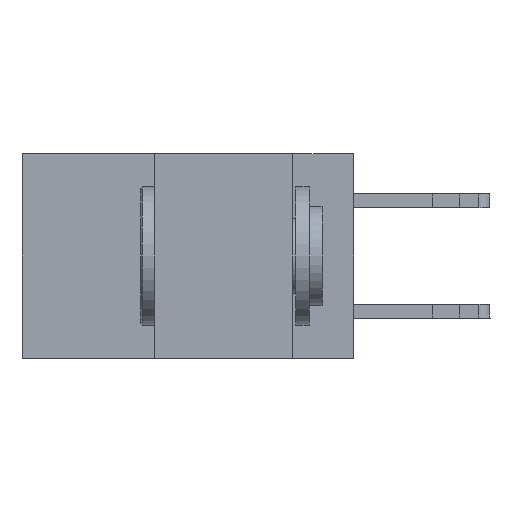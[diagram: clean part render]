
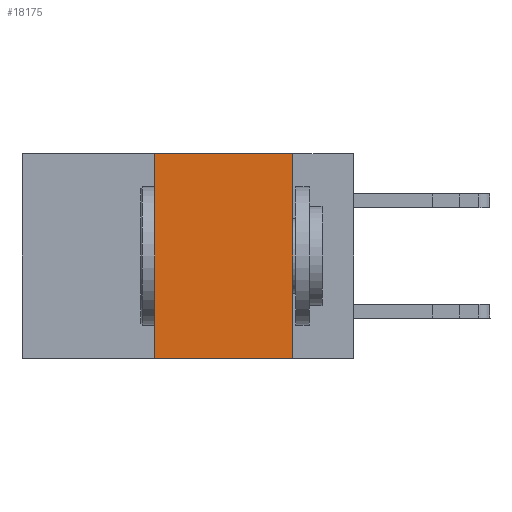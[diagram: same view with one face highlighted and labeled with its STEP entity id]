
A CAD part, left-side view. The second image highlights one B-rep face of the part: STEP entity #18175.
In plain terms, the highlighted planar face has unit normal (-1, 0, 0).
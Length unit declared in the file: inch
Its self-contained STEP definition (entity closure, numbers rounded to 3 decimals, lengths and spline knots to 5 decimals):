
#351 = EDGE_CURVE ( 'NONE', #27454, #6469, #26535, .T. ) ;
#2297 = ORIENTED_EDGE ( 'NONE', *, *, #351, .F. ) ;
#3626 = CARTESIAN_POINT ( 'NONE',  ( 0., 0.11, 0. ) ) ;
#4558 = EDGE_CURVE ( 'NONE', #6469, #20078, #29468, .T. ) ;
#5066 = CARTESIAN_POINT ( 'NONE',  ( 0., 0.36, 0. ) ) ;
#5669 = CARTESIAN_POINT ( 'NONE',  ( 0., 0.11, 0. ) ) ;
#5768 = CARTESIAN_POINT ( 'NONE',  ( 0., 0.6, 0. ) ) ;
#6469 = VERTEX_POINT ( 'NONE', #5669 ) ;
#6593 = LINE ( 'NONE', #22455, #13345 ) ;
#7315 = DIRECTION ( 'NONE',  ( 0., 0., 1. ) ) ;
#8545 = DIRECTION ( 'NONE',  ( 1., 0., 0. ) ) ;
#8877 = DIRECTION ( 'NONE',  ( 0., -1., 0. ) ) ;
#9134 = ORIENTED_EDGE ( 'NONE', *, *, #4558, .F. ) ;
#10263 = ORIENTED_EDGE ( 'NONE', *, *, #30330, .F. ) ;
#10388 = CARTESIAN_POINT ( 'NONE',  ( 0., 0.6, 0. ) ) ;
#10645 = CARTESIAN_POINT ( 'NONE',  ( 0., 0.36, -0.37 ) ) ;
#12871 = VECTOR ( 'NONE', #30540, 39.37008 ) ;
#13345 = VECTOR ( 'NONE', #7315, 39.37008 ) ;
#13580 = VECTOR ( 'NONE', #8877, 39.37008 ) ;
#14417 = DIRECTION ( 'NONE',  ( 0., 0., -1. ) ) ;
#15294 = CARTESIAN_POINT ( 'NONE',  ( 0., 0.11, -0.37 ) ) ;
#15397 = EDGE_LOOP ( 'NONE', ( #9134, #2297, #10263, #31603 ) ) ;
#17015 = EDGE_CURVE ( 'NONE', #22631, #20078, #20775, .T. ) ;
#17770 = AXIS2_PLACEMENT_3D ( 'NONE', #5768, #8545, #26467 ) ;
#17925 = FACE_OUTER_BOUND ( 'NONE', #15397, .T. ) ;
#18175 = ADVANCED_FACE ( 'NONE', ( #17925 ), #21090, .F. ) ;
#20078 = VERTEX_POINT ( 'NONE', #15294 ) ;
#20775 = LINE ( 'NONE', #23538, #13580 ) ;
#21090 = PLANE ( 'NONE',  #17770 ) ;
#21490 = VECTOR ( 'NONE', #14417, 39.37008 ) ;
#22455 = CARTESIAN_POINT ( 'NONE',  ( 0., 0.36, 0. ) ) ;
#22631 = VERTEX_POINT ( 'NONE', #10645 ) ;
#23538 = CARTESIAN_POINT ( 'NONE',  ( 0., 0.6, -0.37 ) ) ;
#26467 = DIRECTION ( 'NONE',  ( 0., 0., -1. ) ) ;
#26535 = LINE ( 'NONE', #10388, #12871 ) ;
#27454 = VERTEX_POINT ( 'NONE', #5066 ) ;
#29468 = LINE ( 'NONE', #3626, #21490 ) ;
#30330 = EDGE_CURVE ( 'NONE', #22631, #27454, #6593, .T. ) ;
#30540 = DIRECTION ( 'NONE',  ( 0., -1., 0. ) ) ;
#31603 = ORIENTED_EDGE ( 'NONE', *, *, #17015, .T. ) ;
